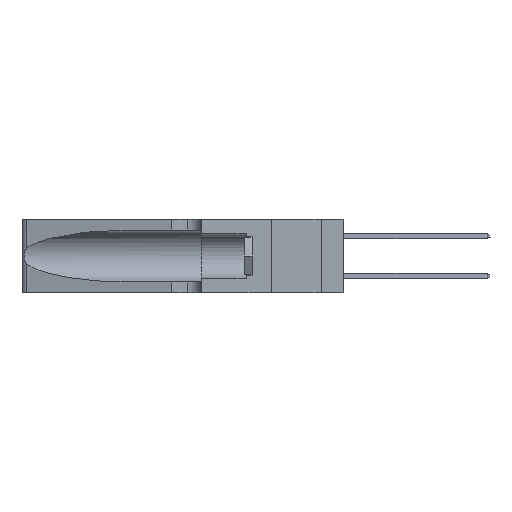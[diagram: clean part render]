
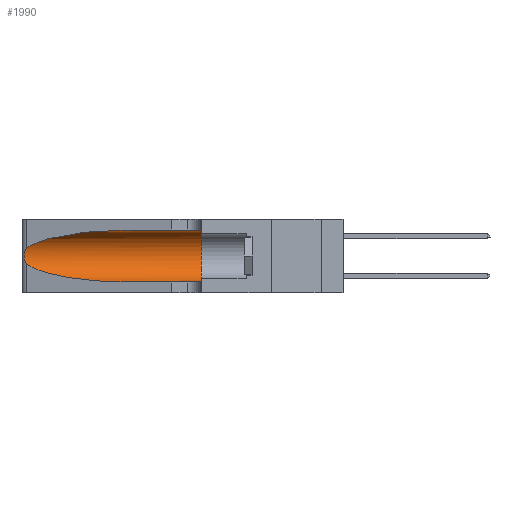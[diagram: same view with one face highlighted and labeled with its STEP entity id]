
A CAD part, left-side view. The second image highlights one B-rep face of the part: STEP entity #1990.
In plain terms, the highlighted cylindrical face has radius 3.308 mm (diameter 6.617 mm), a partial arc.
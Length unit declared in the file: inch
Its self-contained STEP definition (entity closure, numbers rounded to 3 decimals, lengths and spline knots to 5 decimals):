
#21 =( BOUNDED_CURVE ( )  B_SPLINE_CURVE ( 3, ( #14034, #18184, #7912, #22330 ),
 .UNSPECIFIED., .F., .F. ) 
 B_SPLINE_CURVE_WITH_KNOTS ( ( 4, 4 ),
 ( 1.5708, 2.84003 ),
 .UNSPECIFIED. ) 
 CURVE ( )  GEOMETRIC_REPRESENTATION_ITEM ( )  RATIONAL_B_SPLINE_CURVE ( ( 1., 0.87, 0.87, 1. ) ) 
 REPRESENTATION_ITEM ( '' )  );
#1079 = EDGE_CURVE ( 'NONE', #9903, #25096, #9666, .T. ) ;
#1808 = ORIENTED_EDGE ( 'NONE', *, *, #1079, .T. ) ;
#1846 = DIRECTION ( 'NONE',  ( 0., -1., 0. ) ) ;
#1990 = ADVANCED_FACE ( 'NONE', ( #23688 ), #7275, .F. ) ;
#2899 =( BOUNDED_CURVE ( )  B_SPLINE_CURVE ( 3, ( #13220, #25479, #5000, #19438 ),
 .UNSPECIFIED., .F., .T. ) 
 B_SPLINE_CURVE_WITH_KNOTS ( ( 4, 4 ),
 ( 3.44316, 4.71239 ),
 .UNSPECIFIED. ) 
 CURVE ( )  GEOMETRIC_REPRESENTATION_ITEM ( )  RATIONAL_B_SPLINE_CURVE ( ( 1., 0.87, 0.87, 1. ) ) 
 REPRESENTATION_ITEM ( '' )  );
#4231 = LINE ( 'NONE', #24519, #9073 ) ;
#4600 = EDGE_CURVE ( 'NONE', #24396, #19645, #4231, .T. ) ;
#5000 = CARTESIAN_POINT ( 'NONE',  ( 0.18966, 0.96281, 0.05475 ) ) ;
#6026 = DIRECTION ( 'NONE',  ( 0., 0., -1. ) ) ;
#6221 = VECTOR ( 'NONE', #16982, 39.37008 ) ;
#6710 = CARTESIAN_POINT ( 'NONE',  ( 0.25487, 1.22718, 0.22369 ) ) ;
#7275 = CYLINDRICAL_SURFACE ( 'NONE', #11543, 0.13025 ) ;
#7654 = CARTESIAN_POINT ( 'NONE',  ( 0.1305, 0.35, 0.185 ) ) ;
#7660 = CARTESIAN_POINT ( 'NONE',  ( 0.25487, 1.22718, 0.14631 ) ) ;
#7794 = CARTESIAN_POINT ( 'NONE',  ( 0.25639, 1.23186, 0.15144 ) ) ;
#7912 = CARTESIAN_POINT ( 'NONE',  ( 0.2373, 1.15595, 0.28018 ) ) ;
#8117 = CARTESIAN_POINT ( 'NONE',  ( 0.25789, 1.23486, 0.15765 ) ) ;
#8147 = CARTESIAN_POINT ( 'NONE',  ( 0.25856, 1.23593, 0.16098 ) ) ;
#8319 = CARTESIAN_POINT ( 'NONE',  ( 0.26017, 1.23833, 0.17102 ) ) ;
#8376 = CARTESIAN_POINT ( 'NONE',  ( 0.26075, 1.23896, 0.178 ) ) ;
#8408 = CARTESIAN_POINT ( 'NONE',  ( 0.26075, 1.23896, 0.19203 ) ) ;
#8491 = CARTESIAN_POINT ( 'NONE',  ( 0.26018, 1.23835, 0.19895 ) ) ;
#8592 = CARTESIAN_POINT ( 'NONE',  ( 0.25854, 1.2359, 0.20912 ) ) ;
#8781 = CARTESIAN_POINT ( 'NONE',  ( 0.25787, 1.23484, 0.2124 ) ) ;
#8865 = CARTESIAN_POINT ( 'NONE',  ( 0.25639, 1.23184, 0.21858 ) ) ;
#8881 = ORIENTED_EDGE ( 'NONE', *, *, #22952, .T. ) ;
#9073 = VECTOR ( 'NONE', #1846, 39.37008 ) ;
#9666 = B_SPLINE_CURVE_WITH_KNOTS ( 'NONE', 3,
 ( #9764, #12226, #8865, #8781, #8592, #8491, #8408, #8376, #8319, #8147, #8117, #7794, #12135, #7660 ),
 .UNSPECIFIED., .F., .F.,
 ( 4, 2, 2, 2, 2, 2, 4 ),
 ( 0., 0.00027, 0.00053, 0.00107, 0.0016, 0.00187, 0.00214 ),
 .UNSPECIFIED. ) ;
#9690 = ORIENTED_EDGE ( 'NONE', *, *, #4600, .F. ) ;
#9720 = AXIS2_PLACEMENT_3D ( 'NONE', #7654, #22090, #9757 ) ;
#9757 = DIRECTION ( 'NONE',  ( 0., 0., 1. ) ) ;
#9764 = CARTESIAN_POINT ( 'NONE',  ( 0.25487, 1.22718, 0.22369 ) ) ;
#9903 = VERTEX_POINT ( 'NONE', #6710 ) ;
#10663 = EDGE_CURVE ( 'NONE', #24396, #9903, #21, .T. ) ;
#10747 = VERTEX_POINT ( 'NONE', #18461 ) ;
#11543 = AXIS2_PLACEMENT_3D ( 'NONE', #20440, #22504, #6026 ) ;
#11570 = ORIENTED_EDGE ( 'NONE', *, *, #17063, .F. ) ;
#11606 = ORIENTED_EDGE ( 'NONE', *, *, #10663, .T. ) ;
#11713 = LINE ( 'NONE', #23086, #6221 ) ;
#12135 = CARTESIAN_POINT ( 'NONE',  ( 0.25555, 1.22993, 0.14849 ) ) ;
#12226 = CARTESIAN_POINT ( 'NONE',  ( 0.25555, 1.22994, 0.2215 ) ) ;
#12394 = CARTESIAN_POINT ( 'NONE',  ( 0.1305, 0.72297, 0.05475 ) ) ;
#13220 = CARTESIAN_POINT ( 'NONE',  ( 0.25487, 1.22718, 0.14631 ) ) ;
#13410 = ORIENTED_EDGE ( 'NONE', *, *, #23372, .T. ) ;
#13551 = EDGE_LOOP ( 'NONE', ( #11606, #1808, #8881, #13410, #11570, #9690 ) ) ;
#14034 = CARTESIAN_POINT ( 'NONE',  ( 0.1305, 0.72297, 0.31525 ) ) ;
#14171 = CARTESIAN_POINT ( 'NONE',  ( 0.25487, 1.22718, 0.14631 ) ) ;
#16982 = DIRECTION ( 'NONE',  ( 0., -1., 0. ) ) ;
#17063 = EDGE_CURVE ( 'NONE', #19645, #10747, #22011, .T. ) ;
#17817 = CARTESIAN_POINT ( 'NONE',  ( 0.1305, 0.72297, 0.31525 ) ) ;
#18184 = CARTESIAN_POINT ( 'NONE',  ( 0.18966, 0.96281, 0.31525 ) ) ;
#18461 = CARTESIAN_POINT ( 'NONE',  ( 0.1305, 0.35, 0.05475 ) ) ;
#19438 = CARTESIAN_POINT ( 'NONE',  ( 0.1305, 0.72297, 0.05475 ) ) ;
#19645 = VERTEX_POINT ( 'NONE', #25855 ) ;
#20440 = CARTESIAN_POINT ( 'NONE',  ( 0.1305, 1.61858, 0.185 ) ) ;
#22011 = CIRCLE ( 'NONE', #9720, 0.13025 ) ;
#22090 = DIRECTION ( 'NONE',  ( 0., 1., 0. ) ) ;
#22330 = CARTESIAN_POINT ( 'NONE',  ( 0.25487, 1.22718, 0.22369 ) ) ;
#22504 = DIRECTION ( 'NONE',  ( 0., -1., 0. ) ) ;
#22952 = EDGE_CURVE ( 'NONE', #25096, #26336, #2899, .T. ) ;
#23086 = CARTESIAN_POINT ( 'NONE',  ( 0.1305, 1.61858, 0.05475 ) ) ;
#23372 = EDGE_CURVE ( 'NONE', #26336, #10747, #11713, .T. ) ;
#23688 = FACE_OUTER_BOUND ( 'NONE', #13551, .T. ) ;
#24396 = VERTEX_POINT ( 'NONE', #17817 ) ;
#24519 = CARTESIAN_POINT ( 'NONE',  ( 0.1305, 1.61858, 0.31525 ) ) ;
#25096 = VERTEX_POINT ( 'NONE', #14171 ) ;
#25479 = CARTESIAN_POINT ( 'NONE',  ( 0.2373, 1.15595, 0.08982 ) ) ;
#25855 = CARTESIAN_POINT ( 'NONE',  ( 0.1305, 0.35, 0.31525 ) ) ;
#26336 = VERTEX_POINT ( 'NONE', #12394 ) ;
